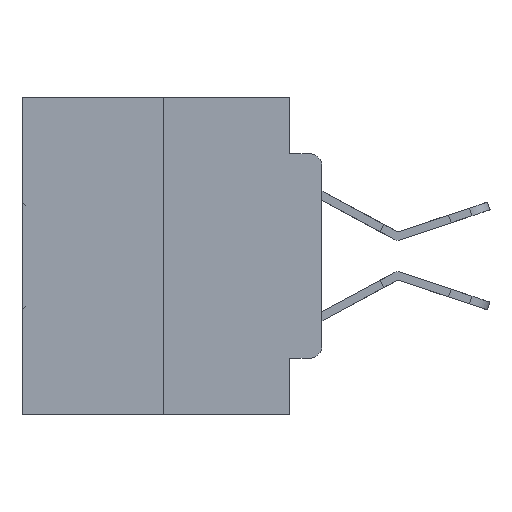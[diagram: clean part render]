
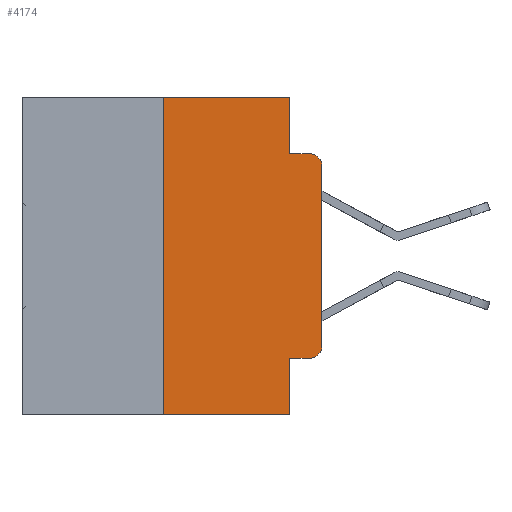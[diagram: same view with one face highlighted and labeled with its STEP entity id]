
A CAD part, left-side view. The second image highlights one B-rep face of the part: STEP entity #4174.
In plain terms, the highlighted planar face has unit normal (-1, 0, 0).
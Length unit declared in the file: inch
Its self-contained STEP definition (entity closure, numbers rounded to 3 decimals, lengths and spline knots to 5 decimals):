
#121 = ORIENTED_EDGE ( 'NONE', *, *, #21607, .F. ) ;
#344 = ORIENTED_EDGE ( 'NONE', *, *, #20347, .F. ) ;
#633 = ORIENTED_EDGE ( 'NONE', *, *, #29535, .T. ) ;
#834 = ORIENTED_EDGE ( 'NONE', *, *, #22525, .F. ) ;
#1115 = ORIENTED_EDGE ( 'NONE', *, *, #18696, .F. ) ;
#1233 = VECTOR ( 'NONE', #5108, 39.37008 ) ;
#1589 = EDGE_CURVE ( 'NONE', #21584, #15628, #27339, .T. ) ;
#1829 = DIRECTION ( 'NONE',  ( 0., 0., -1. ) ) ;
#2038 = ORIENTED_EDGE ( 'NONE', *, *, #8246, .T. ) ;
#2224 = FACE_OUTER_BOUND ( 'NONE', #5842, .T. ) ;
#2364 = DIRECTION ( 'NONE',  ( 0., -1., 0. ) ) ;
#2563 = CARTESIAN_POINT ( 'NONE',  ( 0., 0.051, 0. ) ) ;
#2804 = VECTOR ( 'NONE', #22051, 39.37008 ) ;
#3018 = CIRCLE ( 'NONE', #23157, 0.02 ) ;
#3214 = LINE ( 'NONE', #12641, #28470 ) ;
#3800 = LINE ( 'NONE', #16115, #16255 ) ;
#4174 = ADVANCED_FACE ( 'NONE', ( #2224 ), #10961, .F. ) ;
#4524 = ORIENTED_EDGE ( 'NONE', *, *, #26741, .F. ) ;
#4647 = CARTESIAN_POINT ( 'NONE',  ( 0., 0.02, -0.4115 ) ) ;
#4693 = ORIENTED_EDGE ( 'NONE', *, *, #16614, .T. ) ;
#4810 = CARTESIAN_POINT ( 'NONE',  ( 0., 0.473, 0. ) ) ;
#4882 = ORIENTED_EDGE ( 'NONE', *, *, #31660, .T. ) ;
#5108 = DIRECTION ( 'NONE',  ( 0., -1., 0. ) ) ;
#5793 = VERTEX_POINT ( 'NONE', #15338 ) ;
#5842 = EDGE_LOOP ( 'NONE', ( #6740, #633, #834, #1115, #121, #344, #2038, #4524, #4693, #4882 ) ) ;
#6740 = ORIENTED_EDGE ( 'NONE', *, *, #1589, .T. ) ;
#6774 = AXIS2_PLACEMENT_3D ( 'NONE', #4810, #26177, #27767 ) ;
#6860 = CARTESIAN_POINT ( 'NONE',  ( 0., 0.051, -0.5 ) ) ;
#8246 = EDGE_CURVE ( 'NONE', #8851, #25347, #21395, .T. ) ;
#8738 = DIRECTION ( 'NONE',  ( 0., -1., 0. ) ) ;
#8851 = VERTEX_POINT ( 'NONE', #9975 ) ;
#9415 = AXIS2_PLACEMENT_3D ( 'NONE', #10918, #27890, #13430 ) ;
#9975 = CARTESIAN_POINT ( 'NONE',  ( 0., 0.25, -0.5 ) ) ;
#10109 = VERTEX_POINT ( 'NONE', #17749 ) ;
#10117 = CARTESIAN_POINT ( 'NONE',  ( 0., 0.473, -0.5 ) ) ;
#10570 = CARTESIAN_POINT ( 'NONE',  ( 0., 0.25, 0. ) ) ;
#10898 = VERTEX_POINT ( 'NONE', #10570 ) ;
#10918 = CARTESIAN_POINT ( 'NONE',  ( 0., 0.02, -0.1085 ) ) ;
#10961 = PLANE ( 'NONE',  #6774 ) ;
#11081 = CARTESIAN_POINT ( 'NONE',  ( 0., 0., -0.3915 ) ) ;
#11329 = CARTESIAN_POINT ( 'NONE',  ( 0., 0.051, -0.0885 ) ) ;
#11898 = VECTOR ( 'NONE', #28103, 39.37008 ) ;
#12604 = DIRECTION ( 'NONE',  ( 0., -1., 0. ) ) ;
#12641 = CARTESIAN_POINT ( 'NONE',  ( 0., 0.051, 0. ) ) ;
#12740 = VECTOR ( 'NONE', #2364, 39.37008 ) ;
#13430 = DIRECTION ( 'NONE',  ( 0., 0., -1. ) ) ;
#14784 = CARTESIAN_POINT ( 'NONE',  ( 0., 0.051, -0.4115 ) ) ;
#14979 = CARTESIAN_POINT ( 'NONE',  ( 0., 0.051, 0. ) ) ;
#15318 = LINE ( 'NONE', #17429, #1233 ) ;
#15338 = CARTESIAN_POINT ( 'NONE',  ( 0., 0.051, -0.4115 ) ) ;
#15384 = VECTOR ( 'NONE', #8738, 39.37008 ) ;
#15628 = VERTEX_POINT ( 'NONE', #25830 ) ;
#16035 = CARTESIAN_POINT ( 'NONE',  ( 0., 0.473, 0. ) ) ;
#16115 = CARTESIAN_POINT ( 'NONE',  ( 0., 0.25, 0. ) ) ;
#16255 = VECTOR ( 'NONE', #30518, 39.37008 ) ;
#16614 = EDGE_CURVE ( 'NONE', #5793, #31096, #26379, .T. ) ;
#16754 = DIRECTION ( 'NONE',  ( -1., 0., 0. ) ) ;
#17429 = CARTESIAN_POINT ( 'NONE',  ( 0., 0.051, -0.0885 ) ) ;
#17749 = CARTESIAN_POINT ( 'NONE',  ( 0., 0.02, -0.0885 ) ) ;
#18437 = LINE ( 'NONE', #14979, #11898 ) ;
#18696 = EDGE_CURVE ( 'NONE', #19201, #23956, #3214, .T. ) ;
#19201 = VERTEX_POINT ( 'NONE', #2563 ) ;
#19811 = CIRCLE ( 'NONE', #9415, 0.02 ) ;
#20347 = EDGE_CURVE ( 'NONE', #8851, #10898, #3800, .T. ) ;
#21395 = LINE ( 'NONE', #10117, #27011 ) ;
#21584 = VERTEX_POINT ( 'NONE', #11081 ) ;
#21607 = EDGE_CURVE ( 'NONE', #10898, #19201, #21830, .T. ) ;
#21830 = LINE ( 'NONE', #16035, #15384 ) ;
#22007 = CARTESIAN_POINT ( 'NONE',  ( 0., 0., 0. ) ) ;
#22051 = DIRECTION ( 'NONE',  ( 0., 0., 1. ) ) ;
#22525 = EDGE_CURVE ( 'NONE', #23956, #10109, #15318, .T. ) ;
#23157 = AXIS2_PLACEMENT_3D ( 'NONE', #31127, #16754, #1829 ) ;
#23956 = VERTEX_POINT ( 'NONE', #11329 ) ;
#24845 = DIRECTION ( 'NONE',  ( 0., 0., -1. ) ) ;
#25347 = VERTEX_POINT ( 'NONE', #6860 ) ;
#25830 = CARTESIAN_POINT ( 'NONE',  ( 0., 0., -0.1085 ) ) ;
#26177 = DIRECTION ( 'NONE',  ( 1., 0., 0. ) ) ;
#26379 = LINE ( 'NONE', #14784, #12740 ) ;
#26741 = EDGE_CURVE ( 'NONE', #5793, #25347, #18437, .T. ) ;
#27011 = VECTOR ( 'NONE', #12604, 39.37008 ) ;
#27339 = LINE ( 'NONE', #22007, #2804 ) ;
#27767 = DIRECTION ( 'NONE',  ( 0., 0., -1. ) ) ;
#27890 = DIRECTION ( 'NONE',  ( -1., 0., 0. ) ) ;
#28103 = DIRECTION ( 'NONE',  ( 0., 0., -1. ) ) ;
#28470 = VECTOR ( 'NONE', #24845, 39.37008 ) ;
#29535 = EDGE_CURVE ( 'NONE', #15628, #10109, #19811, .T. ) ;
#30518 = DIRECTION ( 'NONE',  ( 0., 0., 1. ) ) ;
#31096 = VERTEX_POINT ( 'NONE', #4647 ) ;
#31127 = CARTESIAN_POINT ( 'NONE',  ( 0., 0.02, -0.3915 ) ) ;
#31660 = EDGE_CURVE ( 'NONE', #31096, #21584, #3018, .T. ) ;
